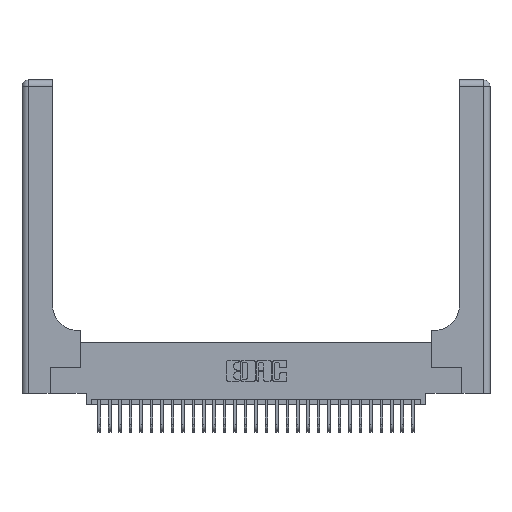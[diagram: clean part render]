
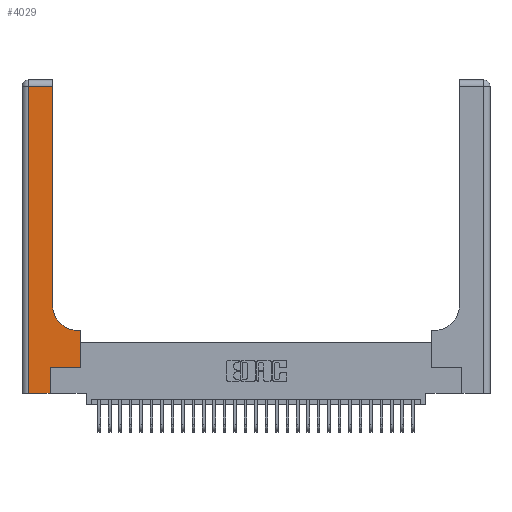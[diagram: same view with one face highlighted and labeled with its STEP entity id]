
A CAD part, top view. The second image highlights one B-rep face of the part: STEP entity #4029.
In plain terms, the highlighted planar face has unit normal (0, 0, 1).
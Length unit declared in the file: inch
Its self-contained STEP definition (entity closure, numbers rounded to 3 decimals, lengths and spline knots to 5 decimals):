
#380 = EDGE_CURVE ( 'NONE', #20007, #23382, #13132, .T. ) ;
#965 = DIRECTION ( 'NONE',  ( 0., -1., 0. ) ) ;
#1091 = EDGE_CURVE ( 'NONE', #27838, #6087, #24303, .T. ) ;
#1347 = CARTESIAN_POINT ( 'NONE',  ( 0.5415, 0.6, 0.37 ) ) ;
#2795 = VECTOR ( 'NONE', #20918, 39.37008 ) ;
#3519 = LINE ( 'NONE', #18603, #2795 ) ;
#3716 = VECTOR ( 'NONE', #24292, 39.37008 ) ;
#3970 = EDGE_LOOP ( 'NONE', ( #17728, #16735, #24022, #10340, #10328, #6402, #15993, #10885, #19027 ) ) ;
#4029 = ADVANCED_FACE ( 'NONE', ( #20064 ), #5119, .F. ) ;
#4654 = VERTEX_POINT ( 'NONE', #26063 ) ;
#5119 = PLANE ( 'NONE',  #11292 ) ;
#5851 = VECTOR ( 'NONE', #8487, 39.37008 ) ;
#6087 = VERTEX_POINT ( 'NONE', #22129 ) ;
#6230 = DIRECTION ( 'NONE',  ( 0., 1., 0. ) ) ;
#6402 = ORIENTED_EDGE ( 'NONE', *, *, #8043, .T. ) ;
#6874 = VECTOR ( 'NONE', #26478, 39.37008 ) ;
#7932 = DIRECTION ( 'NONE',  ( -1., 0., 0. ) ) ;
#8043 = EDGE_CURVE ( 'NONE', #23382, #4654, #16258, .T. ) ;
#8487 = DIRECTION ( 'NONE',  ( 0., 1., 0. ) ) ;
#9285 = VECTOR ( 'NONE', #24961, 39.37008 ) ;
#10328 = ORIENTED_EDGE ( 'NONE', *, *, #380, .T. ) ;
#10340 = ORIENTED_EDGE ( 'NONE', *, *, #26598, .T. ) ;
#10885 = ORIENTED_EDGE ( 'NONE', *, *, #21405, .T. ) ;
#11292 = AXIS2_PLACEMENT_3D ( 'NONE', #28349, #12211, #28453 ) ;
#11544 = DIRECTION ( 'NONE',  ( 0., 0., -1. ) ) ;
#11708 = VERTEX_POINT ( 'NONE', #19102 ) ;
#12177 = EDGE_CURVE ( 'NONE', #26711, #11708, #15315, .T. ) ;
#12211 = DIRECTION ( 'NONE',  ( 0., 0., -1. ) ) ;
#13132 = LINE ( 'NONE', #19212, #6874 ) ;
#13855 = CARTESIAN_POINT ( 'NONE',  ( 0.5585, 0.6, 0.37 ) ) ;
#15315 = CIRCLE ( 'NONE', #20758, 0.25 ) ;
#15446 = CARTESIAN_POINT ( 'NONE',  ( 0.2915, 3., 0.37 ) ) ;
#15993 = ORIENTED_EDGE ( 'NONE', *, *, #27443, .T. ) ;
#16246 = CARTESIAN_POINT ( 'NONE',  ( 0.06, 2.94, 0.37 ) ) ;
#16258 = LINE ( 'NONE', #22628, #9285 ) ;
#16735 = ORIENTED_EDGE ( 'NONE', *, *, #20804, .T. ) ;
#16843 = CARTESIAN_POINT ( 'NONE',  ( 0., 0., 0.37 ) ) ;
#16922 = LINE ( 'NONE', #16843, #3716 ) ;
#17269 = CARTESIAN_POINT ( 'NONE',  ( 0.2915, 0.6, 0.37 ) ) ;
#17728 = ORIENTED_EDGE ( 'NONE', *, *, #27411, .T. ) ;
#18167 = VECTOR ( 'NONE', #965, 39.37008 ) ;
#18603 = CARTESIAN_POINT ( 'NONE',  ( 0., 2.94, 0.37 ) ) ;
#19027 = ORIENTED_EDGE ( 'NONE', *, *, #12177, .T. ) ;
#19102 = CARTESIAN_POINT ( 'NONE',  ( 0.2915, 0.85, 0.37 ) ) ;
#19212 = CARTESIAN_POINT ( 'NONE',  ( 0.269, 0., 0.37 ) ) ;
#20007 = VERTEX_POINT ( 'NONE', #20453 ) ;
#20064 = FACE_OUTER_BOUND ( 'NONE', #3970, .T. ) ;
#20199 = CARTESIAN_POINT ( 'NONE',  ( 0.5585, 0.25, 0.37 ) ) ;
#20234 = CARTESIAN_POINT ( 'NONE',  ( 0.269, 0.25, 0.37 ) ) ;
#20453 = CARTESIAN_POINT ( 'NONE',  ( 0.269, 0., 0.37 ) ) ;
#20758 = AXIS2_PLACEMENT_3D ( 'NONE', #25447, #11544, #27800 ) ;
#20804 = EDGE_CURVE ( 'NONE', #29981, #27838, #3519, .T. ) ;
#20918 = DIRECTION ( 'NONE',  ( -1., 0., 0. ) ) ;
#21405 = EDGE_CURVE ( 'NONE', #28907, #26711, #25350, .T. ) ;
#22129 = CARTESIAN_POINT ( 'NONE',  ( 0.06, 0., 0.37 ) ) ;
#22628 = CARTESIAN_POINT ( 'NONE',  ( 0.269, 0.25, 0.37 ) ) ;
#23382 = VERTEX_POINT ( 'NONE', #20234 ) ;
#23724 = LINE ( 'NONE', #20199, #29914 ) ;
#23909 = VECTOR ( 'NONE', #7932, 39.37008 ) ;
#24022 = ORIENTED_EDGE ( 'NONE', *, *, #1091, .T. ) ;
#24292 = DIRECTION ( 'NONE',  ( 1., 0., 0. ) ) ;
#24303 = LINE ( 'NONE', #26551, #18167 ) ;
#24433 = LINE ( 'NONE', #15446, #5851 ) ;
#24507 = CARTESIAN_POINT ( 'NONE',  ( 0.2915, 2.94, 0.37 ) ) ;
#24961 = DIRECTION ( 'NONE',  ( 1., 0., 0. ) ) ;
#25350 = LINE ( 'NONE', #17269, #23909 ) ;
#25447 = CARTESIAN_POINT ( 'NONE',  ( 0.5415, 0.85, 0.37 ) ) ;
#26063 = CARTESIAN_POINT ( 'NONE',  ( 0.5585, 0.25, 0.37 ) ) ;
#26478 = DIRECTION ( 'NONE',  ( 0., 1., 0. ) ) ;
#26551 = CARTESIAN_POINT ( 'NONE',  ( 0.06, 3., 0.37 ) ) ;
#26598 = EDGE_CURVE ( 'NONE', #6087, #20007, #16922, .T. ) ;
#26711 = VERTEX_POINT ( 'NONE', #1347 ) ;
#27411 = EDGE_CURVE ( 'NONE', #11708, #29981, #24433, .T. ) ;
#27443 = EDGE_CURVE ( 'NONE', #4654, #28907, #23724, .T. ) ;
#27800 = DIRECTION ( 'NONE',  ( 1., 0., 0. ) ) ;
#27838 = VERTEX_POINT ( 'NONE', #16246 ) ;
#28349 = CARTESIAN_POINT ( 'NONE',  ( 0., 3., 0.37 ) ) ;
#28453 = DIRECTION ( 'NONE',  ( -1., 0., 0. ) ) ;
#28907 = VERTEX_POINT ( 'NONE', #13855 ) ;
#29914 = VECTOR ( 'NONE', #6230, 39.37008 ) ;
#29981 = VERTEX_POINT ( 'NONE', #24507 ) ;
